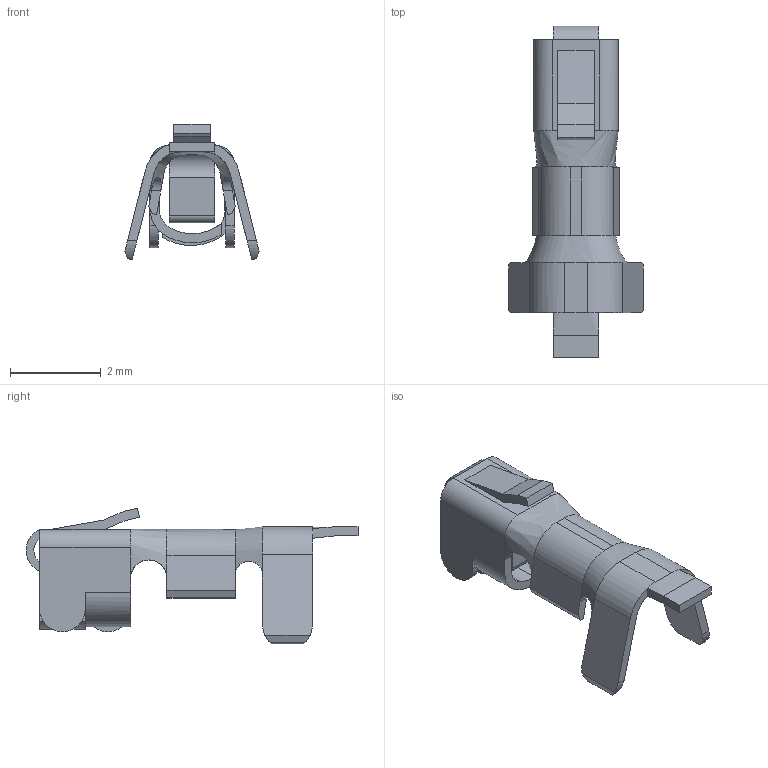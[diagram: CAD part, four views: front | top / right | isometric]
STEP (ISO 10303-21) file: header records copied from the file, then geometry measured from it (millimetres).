
FILE_DESCRIPTION (( 'STEP AP203' ), '1' );
FILE_NAME ('14K-292-452.STEP', '2024-02-22T15:10:14', ( '' ), ( '' ), 'SwSTEP 2.0', 'SolidWorks 2023', '' );
FILE_SCHEMA (( 'CONFIG_CONTROL_DESIGN' ));
Length unit declared in the file: millimetre
Products named in the file (1): 14K-292-452
Bounding box: 2.95 x 7.3 x 2.98 mm (x, y, z)
Volume: 6.8 mm3; surface area: 78.4 mm2
Topology: 1 solids, 1 shells, 116 faces, 329 edges, 214 vertices
Faces by surface type: plane 69, cylinder 37, bspline 10
Entity records: 4274 total; most frequent: CARTESIAN_POINT 1249, ORIENTED_EDGE 658, DIRECTION 570, EDGE_CURVE 329, LINE 218, VECTOR 218, VERTEX_POINT 214, AXIS2_PLACEMENT_3D 176
